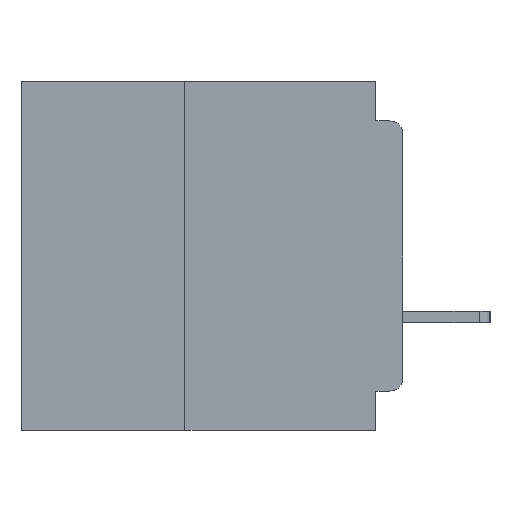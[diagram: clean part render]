
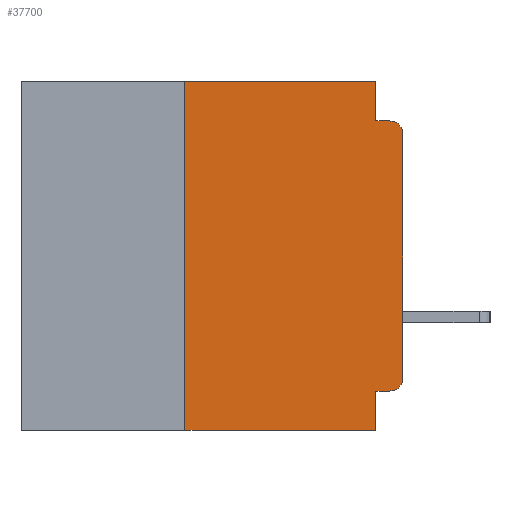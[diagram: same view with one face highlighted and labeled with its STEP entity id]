
A CAD part, left-side view. The second image highlights one B-rep face of the part: STEP entity #37700.
In plain terms, the highlighted planar face has unit normal (-1, 0, 0).
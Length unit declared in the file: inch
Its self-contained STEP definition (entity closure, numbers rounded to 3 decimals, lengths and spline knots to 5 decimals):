
#238 = DIRECTION ( 'NONE',  ( 0., 0., -1. ) ) ;
#309 = CARTESIAN_POINT ( 'NONE',  ( 0., 0.031, -0.045 ) ) ;
#641 = VECTOR ( 'NONE', #16619, 39.37008 ) ;
#852 = AXIS2_PLACEMENT_3D ( 'NONE', #29695, #6206, #33624 ) ;
#879 = DIRECTION ( 'NONE',  ( 0., 0., 1. ) ) ;
#1309 = VECTOR ( 'NONE', #34503, 39.37008 ) ;
#1856 = CARTESIAN_POINT ( 'NONE',  ( 0., 0., -0.045 ) ) ;
#2557 = LINE ( 'NONE', #49962, #22146 ) ;
#3140 = DIRECTION ( 'NONE',  ( 0., 1., 0. ) ) ;
#4080 = CARTESIAN_POINT ( 'NONE',  ( 0., 0.015, -0.06 ) ) ;
#6206 = DIRECTION ( 'NONE',  ( 1., 0., 0. ) ) ;
#7401 = ORIENTED_EDGE ( 'NONE', *, *, #7913, .T. ) ;
#7913 = EDGE_CURVE ( 'NONE', #17251, #13486, #27821, .T. ) ;
#7957 = DIRECTION ( 'NONE',  ( 0., 0., -1. ) ) ;
#8097 = EDGE_LOOP ( 'NONE', ( #14540, #7401, #41497, #35870, #28688, #34787, #28127, #18634, #33904, #22283 ) ) ;
#9478 = VERTEX_POINT ( 'NONE', #49673 ) ;
#9954 = CARTESIAN_POINT ( 'NONE',  ( 0., 0.031, 0. ) ) ;
#10248 = LINE ( 'NONE', #1856, #50576 ) ;
#10261 = LINE ( 'NONE', #18521, #40288 ) ;
#11056 = LINE ( 'NONE', #40101, #641 ) ;
#11604 = LINE ( 'NONE', #31586, #22047 ) ;
#13486 = VERTEX_POINT ( 'NONE', #17612 ) ;
#13775 = EDGE_CURVE ( 'NONE', #26955, #39301, #47822, .T. ) ;
#14540 = ORIENTED_EDGE ( 'NONE', *, *, #14580, .T. ) ;
#14580 = EDGE_CURVE ( 'NONE', #39301, #17251, #11056, .T. ) ;
#16619 = DIRECTION ( 'NONE',  ( 0., 0., 1. ) ) ;
#17251 = VERTEX_POINT ( 'NONE', #39557 ) ;
#17612 = CARTESIAN_POINT ( 'NONE',  ( 0., 0.015, -0.045 ) ) ;
#17663 = FACE_OUTER_BOUND ( 'NONE', #8097, .T. ) ;
#17839 = PLANE ( 'NONE',  #852 ) ;
#18521 = CARTESIAN_POINT ( 'NONE',  ( 0., 0.031, 0. ) ) ;
#18634 = ORIENTED_EDGE ( 'NONE', *, *, #36681, .F. ) ;
#18728 = EDGE_CURVE ( 'NONE', #34984, #9478, #21319, .T. ) ;
#18956 = EDGE_CURVE ( 'NONE', #37004, #49601, #10261, .T. ) ;
#19353 = CARTESIAN_POINT ( 'NONE',  ( 0., 0.437, 0. ) ) ;
#20066 = VECTOR ( 'NONE', #879, 39.37008 ) ;
#20388 = CARTESIAN_POINT ( 'NONE',  ( 0., 0.25, -0.4 ) ) ;
#20495 = VERTEX_POINT ( 'NONE', #36536 ) ;
#21207 = AXIS2_PLACEMENT_3D ( 'NONE', #23391, #50684, #27337 ) ;
#21319 = LINE ( 'NONE', #20388, #20066 ) ;
#22047 = VECTOR ( 'NONE', #238, 39.37008 ) ;
#22146 = VECTOR ( 'NONE', #3140, 39.37008 ) ;
#22283 = ORIENTED_EDGE ( 'NONE', *, *, #13775, .T. ) ;
#23391 = CARTESIAN_POINT ( 'NONE',  ( 0., 0.015, -0.34 ) ) ;
#23460 = DIRECTION ( 'NONE',  ( 0., -1., 0. ) ) ;
#24036 = CARTESIAN_POINT ( 'NONE',  ( 0., 0.25, -0.4 ) ) ;
#24937 = EDGE_CURVE ( 'NONE', #9478, #37004, #43229, .T. ) ;
#25259 = AXIS2_PLACEMENT_3D ( 'NONE', #4080, #31463, #7957 ) ;
#26955 = VERTEX_POINT ( 'NONE', #28953 ) ;
#27337 = DIRECTION ( 'NONE',  ( 0., 0., -1. ) ) ;
#27706 = CARTESIAN_POINT ( 'NONE',  ( 0., 0.031, -0.4 ) ) ;
#27821 = CIRCLE ( 'NONE', #25259, 0.015 ) ;
#28127 = ORIENTED_EDGE ( 'NONE', *, *, #42096, .T. ) ;
#28688 = ORIENTED_EDGE ( 'NONE', *, *, #24937, .F. ) ;
#28953 = CARTESIAN_POINT ( 'NONE',  ( 0., 0.015, -0.355 ) ) ;
#29695 = CARTESIAN_POINT ( 'NONE',  ( 0., 0.437, 0. ) ) ;
#30555 = CARTESIAN_POINT ( 'NONE',  ( 0., 0.437, -0.4 ) ) ;
#31463 = DIRECTION ( 'NONE',  ( -1., 0., 0. ) ) ;
#31586 = CARTESIAN_POINT ( 'NONE',  ( 0., 0.031, -0.4 ) ) ;
#32599 = LINE ( 'NONE', #30555, #1309 ) ;
#33624 = DIRECTION ( 'NONE',  ( 0., 0., -1. ) ) ;
#33904 = ORIENTED_EDGE ( 'NONE', *, *, #42092, .F. ) ;
#34503 = DIRECTION ( 'NONE',  ( 0., -1., 0. ) ) ;
#34787 = ORIENTED_EDGE ( 'NONE', *, *, #18728, .F. ) ;
#34984 = VERTEX_POINT ( 'NONE', #24036 ) ;
#35870 = ORIENTED_EDGE ( 'NONE', *, *, #18956, .F. ) ;
#36207 = CARTESIAN_POINT ( 'NONE',  ( 0., 0., -0.34 ) ) ;
#36536 = CARTESIAN_POINT ( 'NONE',  ( 0., 0.031, -0.355 ) ) ;
#36681 = EDGE_CURVE ( 'NONE', #20495, #42940, #11604, .T. ) ;
#37004 = VERTEX_POINT ( 'NONE', #9954 ) ;
#37160 = DIRECTION ( 'NONE',  ( 0., -1., 0. ) ) ;
#37700 = ADVANCED_FACE ( 'NONE', ( #17663 ), #17839, .F. ) ;
#38318 = EDGE_CURVE ( 'NONE', #49601, #13486, #10248, .T. ) ;
#39301 = VERTEX_POINT ( 'NONE', #36207 ) ;
#39557 = CARTESIAN_POINT ( 'NONE',  ( 0., 0., -0.06 ) ) ;
#40101 = CARTESIAN_POINT ( 'NONE',  ( 0., 0., 0. ) ) ;
#40288 = VECTOR ( 'NONE', #46017, 39.37008 ) ;
#40825 = VECTOR ( 'NONE', #23460, 39.37008 ) ;
#41497 = ORIENTED_EDGE ( 'NONE', *, *, #38318, .F. ) ;
#42092 = EDGE_CURVE ( 'NONE', #26955, #20495, #2557, .T. ) ;
#42096 = EDGE_CURVE ( 'NONE', #34984, #42940, #32599, .T. ) ;
#42940 = VERTEX_POINT ( 'NONE', #27706 ) ;
#43229 = LINE ( 'NONE', #19353, #40825 ) ;
#46017 = DIRECTION ( 'NONE',  ( 0., 0., -1. ) ) ;
#47822 = CIRCLE ( 'NONE', #21207, 0.015 ) ;
#49601 = VERTEX_POINT ( 'NONE', #309 ) ;
#49673 = CARTESIAN_POINT ( 'NONE',  ( 0., 0.25, 0. ) ) ;
#49962 = CARTESIAN_POINT ( 'NONE',  ( 0., 0., -0.355 ) ) ;
#50576 = VECTOR ( 'NONE', #37160, 39.37008 ) ;
#50684 = DIRECTION ( 'NONE',  ( -1., 0., 0. ) ) ;
